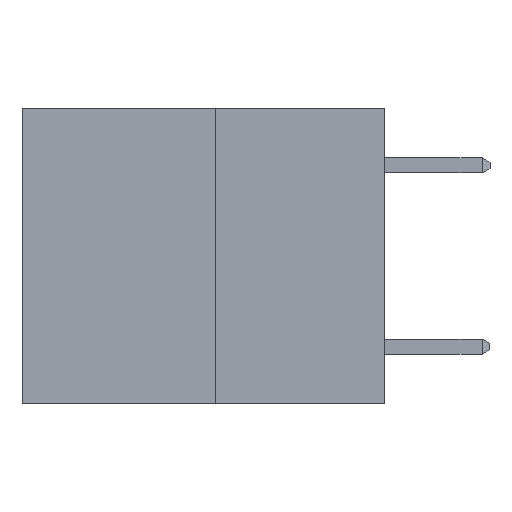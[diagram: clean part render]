
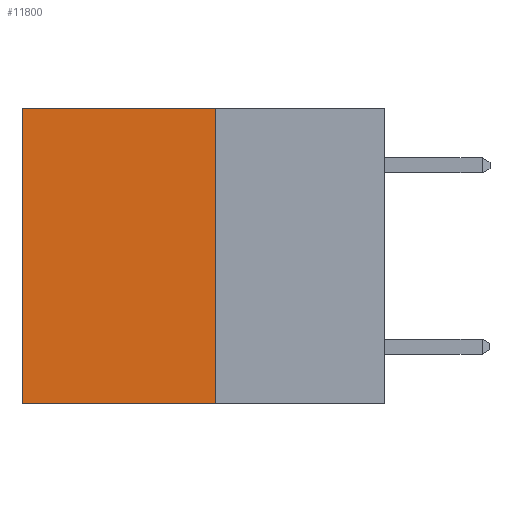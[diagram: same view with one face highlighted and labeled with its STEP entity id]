
A CAD part, left-side view. The second image highlights one B-rep face of the part: STEP entity #11800.
In plain terms, the highlighted planar face has unit normal (-1, 0, 0).
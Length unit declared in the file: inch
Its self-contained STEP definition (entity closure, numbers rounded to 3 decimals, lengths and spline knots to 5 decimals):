
#821 = DIRECTION ( 'NONE',  ( 0., 0., -1. ) ) ;
#1230 = ORIENTED_EDGE ( 'NONE', *, *, #1848, .F. ) ;
#1573 = VERTEX_POINT ( 'NONE', #12234 ) ;
#1848 = EDGE_CURVE ( 'NONE', #7041, #12118, #13486, .T. ) ;
#2038 = ORIENTED_EDGE ( 'NONE', *, *, #13795, .F. ) ;
#2923 = AXIS2_PLACEMENT_3D ( 'NONE', #7439, #13440, #6188 ) ;
#3765 = CARTESIAN_POINT ( 'NONE',  ( 0.3165, 0.28, -0.49 ) ) ;
#4218 = CARTESIAN_POINT ( 'NONE',  ( 0.3165, 0.28, -0.49 ) ) ;
#4325 = CARTESIAN_POINT ( 'NONE',  ( 0.3165, 0.6, -0.49 ) ) ;
#4824 = VECTOR ( 'NONE', #12478, 39.37008 ) ;
#5206 = EDGE_CURVE ( 'NONE', #7478, #12118, #7485, .T. ) ;
#5211 = CARTESIAN_POINT ( 'NONE',  ( 0.3165, 0.6, 0. ) ) ;
#5514 = LINE ( 'NONE', #7722, #11086 ) ;
#6093 = ORIENTED_EDGE ( 'NONE', *, *, #13358, .T. ) ;
#6188 = DIRECTION ( 'NONE',  ( 0., 0., -1. ) ) ;
#6350 = VECTOR ( 'NONE', #821, 39.37008 ) ;
#6415 = CARTESIAN_POINT ( 'NONE',  ( 0.3165, 0.6, -0.49 ) ) ;
#7041 = VERTEX_POINT ( 'NONE', #3765 ) ;
#7439 = CARTESIAN_POINT ( 'NONE',  ( 0.3165, 0.28, -0.49 ) ) ;
#7478 = VERTEX_POINT ( 'NONE', #5211 ) ;
#7485 = LINE ( 'NONE', #4325, #6350 ) ;
#7722 = CARTESIAN_POINT ( 'NONE',  ( 0.3165, 0.28, 0. ) ) ;
#9273 = LINE ( 'NONE', #4218, #4824 ) ;
#9478 = FACE_OUTER_BOUND ( 'NONE', #9745, .T. ) ;
#9745 = EDGE_LOOP ( 'NONE', ( #13406, #1230, #2038, #6093 ) ) ;
#9844 = VECTOR ( 'NONE', #14856, 39.37008 ) ;
#11086 = VECTOR ( 'NONE', #11444, 39.37008 ) ;
#11444 = DIRECTION ( 'NONE',  ( 0., 1., 0. ) ) ;
#11800 = ADVANCED_FACE ( 'NONE', ( #9478 ), #13380, .F. ) ;
#12118 = VERTEX_POINT ( 'NONE', #6415 ) ;
#12234 = CARTESIAN_POINT ( 'NONE',  ( 0.3165, 0.28, 0. ) ) ;
#12478 = DIRECTION ( 'NONE',  ( 0., 0., -1. ) ) ;
#13358 = EDGE_CURVE ( 'NONE', #1573, #7478, #5514, .T. ) ;
#13380 = PLANE ( 'NONE',  #2923 ) ;
#13406 = ORIENTED_EDGE ( 'NONE', *, *, #5206, .T. ) ;
#13440 = DIRECTION ( 'NONE',  ( 1., 0., 0. ) ) ;
#13486 = LINE ( 'NONE', #14595, #9844 ) ;
#13795 = EDGE_CURVE ( 'NONE', #1573, #7041, #9273, .T. ) ;
#14595 = CARTESIAN_POINT ( 'NONE',  ( 0.3165, 0.28, -0.49 ) ) ;
#14856 = DIRECTION ( 'NONE',  ( 0., 1., 0. ) ) ;
